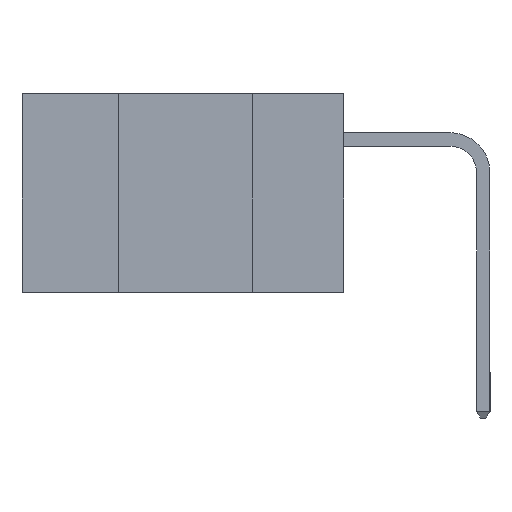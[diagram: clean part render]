
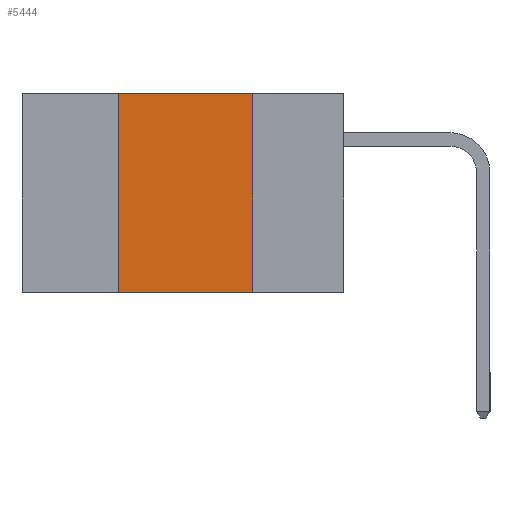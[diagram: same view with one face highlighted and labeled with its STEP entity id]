
A CAD part, left-side view. The second image highlights one B-rep face of the part: STEP entity #5444.
In plain terms, the highlighted planar face has unit normal (-1, 0, 0).
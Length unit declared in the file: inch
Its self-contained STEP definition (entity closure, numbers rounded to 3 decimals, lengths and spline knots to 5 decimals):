
#396 = VECTOR ( 'NONE', #6018, 39.37008 ) ;
#508 = CARTESIAN_POINT ( 'NONE',  ( 0., 0.42, 0. ) ) ;
#1103 = LINE ( 'NONE', #11165, #3719 ) ;
#1302 = EDGE_CURVE ( 'NONE', #9285, #2167, #5973, .T. ) ;
#1441 = DIRECTION ( 'NONE',  ( 1., 0., 0. ) ) ;
#1535 = VERTEX_POINT ( 'NONE', #508 ) ;
#1553 = VECTOR ( 'NONE', #4685, 39.37008 ) ;
#1606 = EDGE_LOOP ( 'NONE', ( #4503, #10938, #4193, #6464 ) ) ;
#2167 = VERTEX_POINT ( 'NONE', #6575 ) ;
#3054 = VECTOR ( 'NONE', #6085, 39.37008 ) ;
#3719 = VECTOR ( 'NONE', #4721, 39.37008 ) ;
#3785 = CARTESIAN_POINT ( 'NONE',  ( 0., 0.17, 0. ) ) ;
#3835 = CARTESIAN_POINT ( 'NONE',  ( 0., 0.6, -0.37 ) ) ;
#4193 = ORIENTED_EDGE ( 'NONE', *, *, #9322, .F. ) ;
#4280 = LINE ( 'NONE', #3785, #1553 ) ;
#4503 = ORIENTED_EDGE ( 'NONE', *, *, #4873, .F. ) ;
#4685 = DIRECTION ( 'NONE',  ( 0., 0., -1. ) ) ;
#4721 = DIRECTION ( 'NONE',  ( 0., -1., 0. ) ) ;
#4873 = EDGE_CURVE ( 'NONE', #7286, #2167, #4280, .T. ) ;
#5001 = CARTESIAN_POINT ( 'NONE',  ( 0., 0.6, 0. ) ) ;
#5255 = CARTESIAN_POINT ( 'NONE',  ( 0., 0.42, 0. ) ) ;
#5444 = ADVANCED_FACE ( 'NONE', ( #8595 ), #5879, .F. ) ;
#5879 = PLANE ( 'NONE',  #6951 ) ;
#5973 = LINE ( 'NONE', #3835, #396 ) ;
#6018 = DIRECTION ( 'NONE',  ( 0., -1., 0. ) ) ;
#6085 = DIRECTION ( 'NONE',  ( 0., 0., 1. ) ) ;
#6464 = ORIENTED_EDGE ( 'NONE', *, *, #1302, .T. ) ;
#6575 = CARTESIAN_POINT ( 'NONE',  ( 0., 0.17, -0.37 ) ) ;
#6951 = AXIS2_PLACEMENT_3D ( 'NONE', #5001, #1441, #8628 ) ;
#7286 = VERTEX_POINT ( 'NONE', #11465 ) ;
#7787 = EDGE_CURVE ( 'NONE', #1535, #7286, #1103, .T. ) ;
#8533 = LINE ( 'NONE', #5255, #3054 ) ;
#8595 = FACE_OUTER_BOUND ( 'NONE', #1606, .T. ) ;
#8628 = DIRECTION ( 'NONE',  ( 0., 0., -1. ) ) ;
#9285 = VERTEX_POINT ( 'NONE', #11442 ) ;
#9322 = EDGE_CURVE ( 'NONE', #9285, #1535, #8533, .T. ) ;
#10938 = ORIENTED_EDGE ( 'NONE', *, *, #7787, .F. ) ;
#11165 = CARTESIAN_POINT ( 'NONE',  ( 0., 0.6, 0. ) ) ;
#11442 = CARTESIAN_POINT ( 'NONE',  ( 0., 0.42, -0.37 ) ) ;
#11465 = CARTESIAN_POINT ( 'NONE',  ( 0., 0.17, 0. ) ) ;
